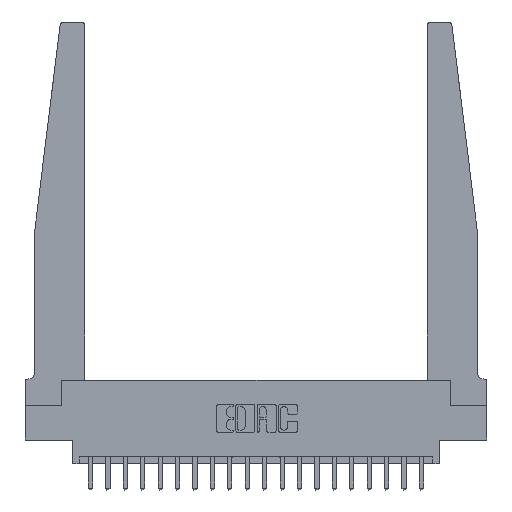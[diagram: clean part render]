
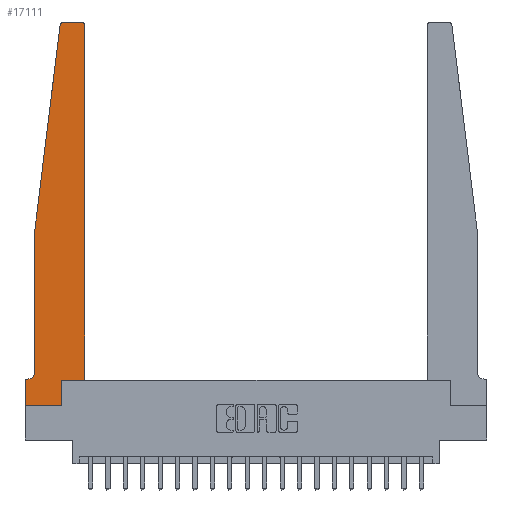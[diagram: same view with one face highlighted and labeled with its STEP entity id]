
A CAD part, top view. The second image highlights one B-rep face of the part: STEP entity #17111.
In plain terms, the highlighted planar face has unit normal (0, 0, 1).
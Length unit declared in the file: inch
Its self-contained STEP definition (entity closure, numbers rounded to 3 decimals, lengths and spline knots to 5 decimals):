
#312 = CARTESIAN_POINT ( 'NONE',  ( 0.065, 0.1875, 0.37 ) ) ;
#447 = VECTOR ( 'NONE', #20210, 39.37008 ) ;
#595 = VERTEX_POINT ( 'NONE', #7974 ) ;
#611 = CARTESIAN_POINT ( 'NONE',  ( 0.015, 0.2375, 0.37 ) ) ;
#815 = DIRECTION ( 'NONE',  ( 0., 0., 1. ) ) ;
#911 = VECTOR ( 'NONE', #13323, 39.37008 ) ;
#1026 = DIRECTION ( 'NONE',  ( 1., 0., 0. ) ) ;
#1049 = LINE ( 'NONE', #2693, #1295 ) ;
#1176 = CIRCLE ( 'NONE', #6748, 0.03 ) ;
#1295 = VECTOR ( 'NONE', #17343, 39.37008 ) ;
#1566 = EDGE_CURVE ( 'NONE', #3265, #17721, #18328, .T. ) ;
#1801 = DIRECTION ( 'NONE',  ( 0., -1., 0. ) ) ;
#1844 = EDGE_CURVE ( 'NONE', #13070, #16412, #9305, .T. ) ;
#2231 = VECTOR ( 'NONE', #12248, 39.37008 ) ;
#2607 = CARTESIAN_POINT ( 'NONE',  ( 0.27653, 2.72, 0.37 ) ) ;
#2693 = CARTESIAN_POINT ( 'NONE',  ( 0., 0., 0.37 ) ) ;
#2971 = EDGE_CURVE ( 'NONE', #17721, #595, #20432, .T. ) ;
#3262 = EDGE_CURVE ( 'NONE', #18954, #14663, #20138, .T. ) ;
#3265 = VERTEX_POINT ( 'NONE', #13607 ) ;
#3572 = AXIS2_PLACEMENT_3D ( 'NONE', #611, #7701, #10850 ) ;
#3771 = EDGE_CURVE ( 'NONE', #16412, #15571, #5672, .T. ) ;
#3796 = CARTESIAN_POINT ( 'NONE',  ( 0.065, 1.25, 0.37 ) ) ;
#4163 = ORIENTED_EDGE ( 'NONE', *, *, #10611, .T. ) ;
#4494 = DIRECTION ( 'NONE',  ( 0., 0., 1. ) ) ;
#4517 = ORIENTED_EDGE ( 'NONE', *, *, #12419, .T. ) ;
#4619 = VERTEX_POINT ( 'NONE', #12507 ) ;
#4651 = VECTOR ( 'NONE', #10467, 39.37008 ) ;
#4959 = VECTOR ( 'NONE', #18908, 39.37008 ) ;
#5240 = VECTOR ( 'NONE', #17016, 39.37008 ) ;
#5312 = EDGE_CURVE ( 'NONE', #20216, #18954, #20387, .T. ) ;
#5564 = DIRECTION ( 'NONE',  ( 0., 0., 1. ) ) ;
#5672 = LINE ( 'NONE', #12282, #4959 ) ;
#6035 = ORIENTED_EDGE ( 'NONE', *, *, #1844, .T. ) ;
#6317 = CARTESIAN_POINT ( 'NONE',  ( 0.2605, 0., 0.37 ) ) ;
#6711 = ORIENTED_EDGE ( 'NONE', *, *, #14180, .T. ) ;
#6748 = AXIS2_PLACEMENT_3D ( 'NONE', #2607, #5564, #12175 ) ;
#7017 = ORIENTED_EDGE ( 'NONE', *, *, #3262, .T. ) ;
#7018 = CARTESIAN_POINT ( 'NONE',  ( 0., 0., 0.37 ) ) ;
#7411 = CARTESIAN_POINT ( 'NONE',  ( 0.2605, 0.18, 0.37 ) ) ;
#7576 = CARTESIAN_POINT ( 'NONE',  ( 0.395, 2.72, 0.37 ) ) ;
#7643 = AXIS2_PLACEMENT_3D ( 'NONE', #9165, #4494, #11115 ) ;
#7701 = DIRECTION ( 'NONE',  ( 0., 0., -1. ) ) ;
#7974 = CARTESIAN_POINT ( 'NONE',  ( 0.395, 2.75, 0.37 ) ) ;
#8029 = ORIENTED_EDGE ( 'NONE', *, *, #11199, .T. ) ;
#8449 = CARTESIAN_POINT ( 'NONE',  ( 0.425, 0.18, 0.37 ) ) ;
#8557 = CARTESIAN_POINT ( 'NONE',  ( 0.425, 0.18, 0.37 ) ) ;
#8940 = VERTEX_POINT ( 'NONE', #18766 ) ;
#9165 = CARTESIAN_POINT ( 'NONE',  ( 0., 0.1875, 0.37 ) ) ;
#9166 = CARTESIAN_POINT ( 'NONE',  ( 0.015, 0.1875, 0.37 ) ) ;
#9305 = LINE ( 'NONE', #15919, #14110 ) ;
#9929 = CARTESIAN_POINT ( 'NONE',  ( 0.24675, 2.72367, 0.37 ) ) ;
#10314 = CARTESIAN_POINT ( 'NONE',  ( 0.065, 1.25, 0.37 ) ) ;
#10467 = DIRECTION ( 'NONE',  ( -1., 0., 0. ) ) ;
#10611 = EDGE_CURVE ( 'NONE', #15571, #3265, #13316, .T. ) ;
#10757 = ORIENTED_EDGE ( 'NONE', *, *, #2971, .T. ) ;
#10850 = DIRECTION ( 'NONE',  ( -1., 0., 0. ) ) ;
#11035 = EDGE_LOOP ( 'NONE', ( #8029, #4517, #15821, #7017, #6711, #15449, #12923, #6035, #19152, #4163, #19738, #10757 ) ) ;
#11115 = DIRECTION ( 'NONE',  ( 1., 0., 0. ) ) ;
#11199 = EDGE_CURVE ( 'NONE', #595, #4619, #19145, .T. ) ;
#11212 = VERTEX_POINT ( 'NONE', #9166 ) ;
#12175 = DIRECTION ( 'NONE',  ( 1., 0., 0. ) ) ;
#12217 = EDGE_CURVE ( 'NONE', #11212, #8940, #15216, .T. ) ;
#12248 = DIRECTION ( 'NONE',  ( -0.122, -0.992, 0. ) ) ;
#12282 = CARTESIAN_POINT ( 'NONE',  ( 0.2605, 0.18, 0.37 ) ) ;
#12419 = EDGE_CURVE ( 'NONE', #4619, #20216, #1176, .T. ) ;
#12507 = CARTESIAN_POINT ( 'NONE',  ( 0.27653, 2.75, 0.37 ) ) ;
#12923 = ORIENTED_EDGE ( 'NONE', *, *, #14128, .T. ) ;
#13070 = VERTEX_POINT ( 'NONE', #7018 ) ;
#13316 = LINE ( 'NONE', #8449, #5240 ) ;
#13323 = DIRECTION ( 'NONE',  ( 0., 1., 0. ) ) ;
#13607 = CARTESIAN_POINT ( 'NONE',  ( 0.425, 0.18, 0.37 ) ) ;
#14110 = VECTOR ( 'NONE', #1026, 39.37008 ) ;
#14128 = EDGE_CURVE ( 'NONE', #8940, #13070, #1049, .T. ) ;
#14180 = EDGE_CURVE ( 'NONE', #14663, #11212, #21208, .T. ) ;
#14663 = VERTEX_POINT ( 'NONE', #20786 ) ;
#15216 = LINE ( 'NONE', #312, #447 ) ;
#15269 = PLANE ( 'NONE',  #7643 ) ;
#15449 = ORIENTED_EDGE ( 'NONE', *, *, #12217, .T. ) ;
#15571 = VERTEX_POINT ( 'NONE', #7411 ) ;
#15821 = ORIENTED_EDGE ( 'NONE', *, *, #5312, .T. ) ;
#15919 = CARTESIAN_POINT ( 'NONE',  ( 0., 0., 0.37 ) ) ;
#16412 = VERTEX_POINT ( 'NONE', #6317 ) ;
#17016 = DIRECTION ( 'NONE',  ( 1., 0., 0. ) ) ;
#17111 = ADVANCED_FACE ( 'NONE', ( #20669 ), #15269, .T. ) ;
#17292 = CARTESIAN_POINT ( 'NONE',  ( 0.25, 2.75, 0.37 ) ) ;
#17343 = DIRECTION ( 'NONE',  ( 0., -1., 0. ) ) ;
#17544 = DIRECTION ( 'NONE',  ( 1., 0., 0. ) ) ;
#17721 = VERTEX_POINT ( 'NONE', #19971 ) ;
#18303 = CARTESIAN_POINT ( 'NONE',  ( 0.065, 1.25, 0.37 ) ) ;
#18328 = LINE ( 'NONE', #8557, #911 ) ;
#18367 = AXIS2_PLACEMENT_3D ( 'NONE', #7576, #815, #17544 ) ;
#18766 = CARTESIAN_POINT ( 'NONE',  ( 0., 0.1875, 0.37 ) ) ;
#18908 = DIRECTION ( 'NONE',  ( 0., 1., 0. ) ) ;
#18954 = VERTEX_POINT ( 'NONE', #10314 ) ;
#19145 = LINE ( 'NONE', #17292, #4651 ) ;
#19152 = ORIENTED_EDGE ( 'NONE', *, *, #3771, .T. ) ;
#19738 = ORIENTED_EDGE ( 'NONE', *, *, #1566, .T. ) ;
#19774 = VECTOR ( 'NONE', #1801, 39.37008 ) ;
#19971 = CARTESIAN_POINT ( 'NONE',  ( 0.425, 2.72, 0.37 ) ) ;
#20138 = LINE ( 'NONE', #18303, #19774 ) ;
#20210 = DIRECTION ( 'NONE',  ( -1., 0., 0. ) ) ;
#20216 = VERTEX_POINT ( 'NONE', #9929 ) ;
#20387 = LINE ( 'NONE', #3796, #2231 ) ;
#20432 = CIRCLE ( 'NONE', #18367, 0.03 ) ;
#20669 = FACE_OUTER_BOUND ( 'NONE', #11035, .T. ) ;
#20786 = CARTESIAN_POINT ( 'NONE',  ( 0.065, 0.2375, 0.37 ) ) ;
#21208 = CIRCLE ( 'NONE', #3572, 0.05 ) ;
